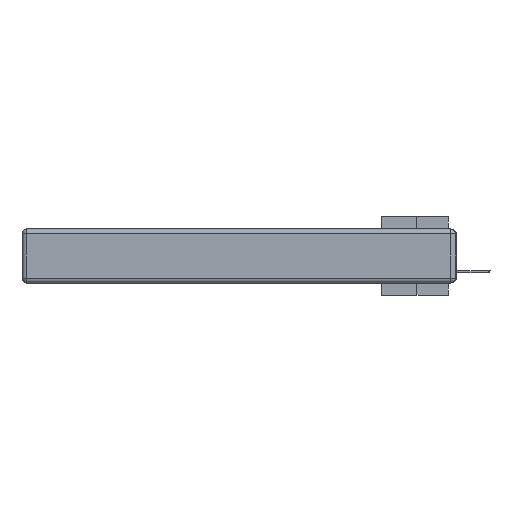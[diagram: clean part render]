
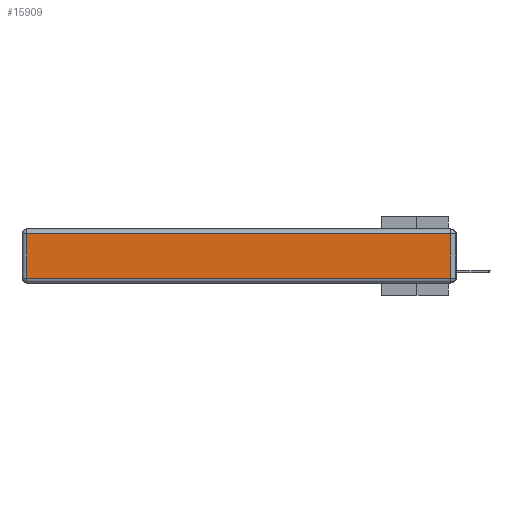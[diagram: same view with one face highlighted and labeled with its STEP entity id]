
A CAD part, left-side view. The second image highlights one B-rep face of the part: STEP entity #15909.
In plain terms, the highlighted planar face has unit normal (-1, 0, 0).
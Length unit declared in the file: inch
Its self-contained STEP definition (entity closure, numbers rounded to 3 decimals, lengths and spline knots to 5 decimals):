
#329 = VECTOR ( 'NONE', #35769, 39.37008 ) ;
#2046 = ORIENTED_EDGE ( 'NONE', *, *, #6299, .T. ) ;
#3018 = DIRECTION ( 'NONE',  ( 0., 0., 1. ) ) ;
#5273 = EDGE_CURVE ( 'NONE', #25585, #19862, #31499, .T. ) ;
#6299 = EDGE_CURVE ( 'NONE', #33801, #25585, #24073, .T. ) ;
#8366 = CARTESIAN_POINT ( 'NONE',  ( 0., 0.03, -0.03 ) ) ;
#8749 = FACE_OUTER_BOUND ( 'NONE', #16434, .T. ) ;
#9201 = LINE ( 'NONE', #21332, #12280 ) ;
#9333 = VECTOR ( 'NONE', #11108, 39.37008 ) ;
#11108 = DIRECTION ( 'NONE',  ( 0., 1., 0. ) ) ;
#12090 = LINE ( 'NONE', #32890, #329 ) ;
#12280 = VECTOR ( 'NONE', #30175, 39.37008 ) ;
#12336 = DIRECTION ( 'NONE',  ( 0., 0., 1. ) ) ;
#12659 = EDGE_CURVE ( 'NONE', #14935, #33801, #12090, .T. ) ;
#13889 = EDGE_CURVE ( 'NONE', #19862, #14935, #9201, .T. ) ;
#14935 = VERTEX_POINT ( 'NONE', #37531 ) ;
#15389 = CARTESIAN_POINT ( 'NONE',  ( 0., 2.72, -0.03 ) ) ;
#15909 = ADVANCED_FACE ( 'NONE', ( #8749 ), #17222, .T. ) ;
#16304 = CARTESIAN_POINT ( 'NONE',  ( 0., 2.75, -0.03 ) ) ;
#16434 = EDGE_LOOP ( 'NONE', ( #36249, #2046, #28638, #33097 ) ) ;
#17103 = VECTOR ( 'NONE', #12336, 39.37008 ) ;
#17222 = PLANE ( 'NONE',  #35976 ) ;
#19862 = VERTEX_POINT ( 'NONE', #15389 ) ;
#21332 = CARTESIAN_POINT ( 'NONE',  ( 0., 2.72, -0.343 ) ) ;
#24073 = LINE ( 'NONE', #35831, #17103 ) ;
#25585 = VERTEX_POINT ( 'NONE', #8366 ) ;
#28638 = ORIENTED_EDGE ( 'NONE', *, *, #5273, .T. ) ;
#29255 = CARTESIAN_POINT ( 'NONE',  ( 0., 0.03, -0.313 ) ) ;
#29333 = DIRECTION ( 'NONE',  ( -1., 0., 0. ) ) ;
#30175 = DIRECTION ( 'NONE',  ( 0., 0., -1. ) ) ;
#31462 = CARTESIAN_POINT ( 'NONE',  ( 0., 0., -0.343 ) ) ;
#31499 = LINE ( 'NONE', #16304, #9333 ) ;
#32890 = CARTESIAN_POINT ( 'NONE',  ( 0., 0., -0.313 ) ) ;
#33097 = ORIENTED_EDGE ( 'NONE', *, *, #13889, .T. ) ;
#33801 = VERTEX_POINT ( 'NONE', #29255 ) ;
#35769 = DIRECTION ( 'NONE',  ( 0., -1., 0. ) ) ;
#35831 = CARTESIAN_POINT ( 'NONE',  ( 0., 0.03, -0.343 ) ) ;
#35976 = AXIS2_PLACEMENT_3D ( 'NONE', #31462, #29333, #3018 ) ;
#36249 = ORIENTED_EDGE ( 'NONE', *, *, #12659, .T. ) ;
#37531 = CARTESIAN_POINT ( 'NONE',  ( 0., 2.72, -0.313 ) ) ;
